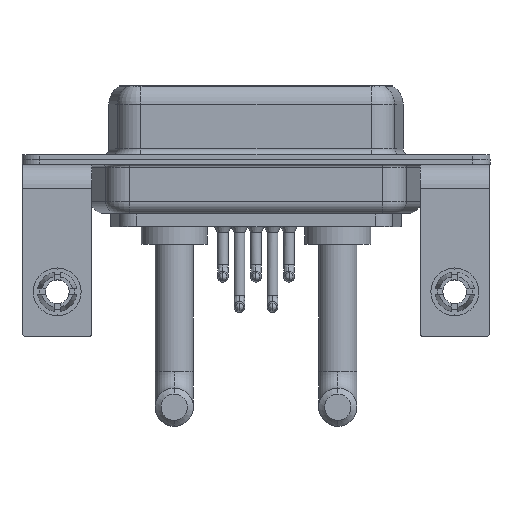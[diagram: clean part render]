
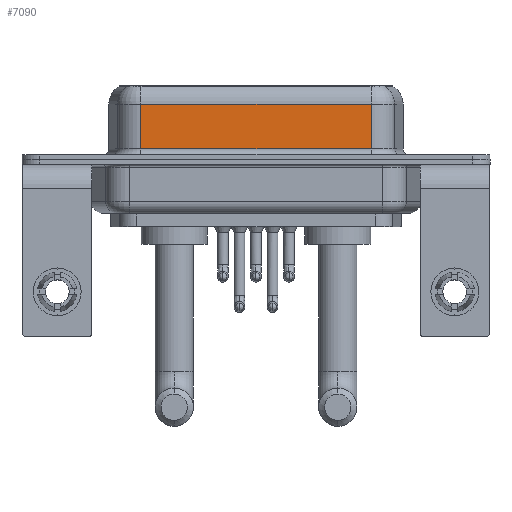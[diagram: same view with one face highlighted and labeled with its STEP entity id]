
A CAD part, front view. The second image highlights one B-rep face of the part: STEP entity #7090.
In plain terms, the highlighted planar face has unit normal (0, -1, 0).
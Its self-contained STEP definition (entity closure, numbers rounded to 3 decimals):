
#788 = VERTEX_POINT ( 'NONE', #4192 ) ;
#936 = VECTOR ( 'NONE', #2401, 1000. ) ;
#1725 = CARTESIAN_POINT ( 'NONE',  ( 7.013, -3.95, 4.65 ) ) ;
#1736 = DIRECTION ( 'NONE',  ( 0., 0., -1. ) ) ;
#1747 = EDGE_LOOP ( 'NONE', ( #10430, #13015, #2854, #12236 ) ) ;
#2242 = DIRECTION ( 'NONE',  ( 1., 0., 0. ) ) ;
#2341 = CARTESIAN_POINT ( 'NONE',  ( 26.287, -3.95, 0.9 ) ) ;
#2401 = DIRECTION ( 'NONE',  ( -1., 0., 0. ) ) ;
#2854 = ORIENTED_EDGE ( 'NONE', *, *, #8108, .T. ) ;
#3176 = CARTESIAN_POINT ( 'NONE',  ( 26.287, -3.95, 6.4 ) ) ;
#3275 = DIRECTION ( 'NONE',  ( 0., 0., 1. ) ) ;
#3346 = CARTESIAN_POINT ( 'NONE',  ( 7.013, -3.95, 6.4 ) ) ;
#4192 = CARTESIAN_POINT ( 'NONE',  ( 26.287, -3.95, 4.65 ) ) ;
#4363 = AXIS2_PLACEMENT_3D ( 'NONE', #3176, #4450, #3275 ) ;
#4450 = DIRECTION ( 'NONE',  ( 0., 1., 0. ) ) ;
#5957 = VECTOR ( 'NONE', #10366, 1000. ) ;
#6090 = PLANE ( 'NONE',  #4363 ) ;
#6810 = EDGE_CURVE ( 'NONE', #788, #18449, #14117, .T. ) ;
#7090 = ADVANCED_FACE ( 'NONE', ( #16529 ), #6090, .F. ) ;
#8108 = EDGE_CURVE ( 'NONE', #18449, #13966, #13396, .T. ) ;
#8165 = CARTESIAN_POINT ( 'NONE',  ( 26.287, -3.95, 0.9 ) ) ;
#8798 = VERTEX_POINT ( 'NONE', #8165 ) ;
#8879 = VECTOR ( 'NONE', #1736, 1000. ) ;
#9148 = LINE ( 'NONE', #15105, #8879 ) ;
#9428 = CARTESIAN_POINT ( 'NONE',  ( 26.287, -3.95, 4.65 ) ) ;
#9644 = LINE ( 'NONE', #2341, #11666 ) ;
#9892 = CARTESIAN_POINT ( 'NONE',  ( 7.013, -3.95, 0.9 ) ) ;
#10366 = DIRECTION ( 'NONE',  ( 0., 0., -1. ) ) ;
#10430 = ORIENTED_EDGE ( 'NONE', *, *, #12194, .F. ) ;
#11666 = VECTOR ( 'NONE', #2242, 1000. ) ;
#11891 = EDGE_CURVE ( 'NONE', #13966, #8798, #9644, .T. ) ;
#12194 = EDGE_CURVE ( 'NONE', #788, #8798, #9148, .T. ) ;
#12236 = ORIENTED_EDGE ( 'NONE', *, *, #11891, .T. ) ;
#13015 = ORIENTED_EDGE ( 'NONE', *, *, #6810, .T. ) ;
#13396 = LINE ( 'NONE', #3346, #5957 ) ;
#13966 = VERTEX_POINT ( 'NONE', #9892 ) ;
#14117 = LINE ( 'NONE', #9428, #936 ) ;
#15105 = CARTESIAN_POINT ( 'NONE',  ( 26.287, -3.95, 6.4 ) ) ;
#16529 = FACE_OUTER_BOUND ( 'NONE', #1747, .T. ) ;
#18449 = VERTEX_POINT ( 'NONE', #1725 ) ;
